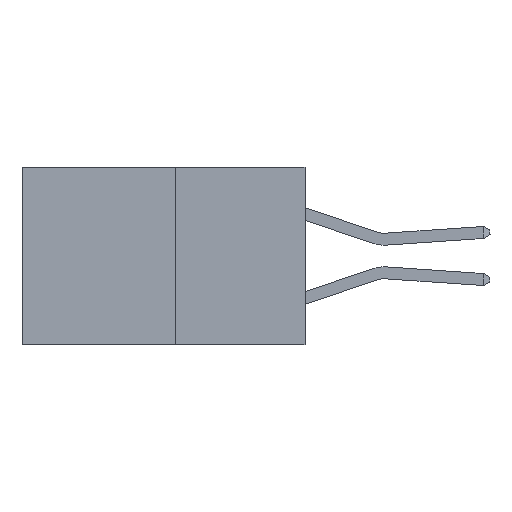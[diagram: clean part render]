
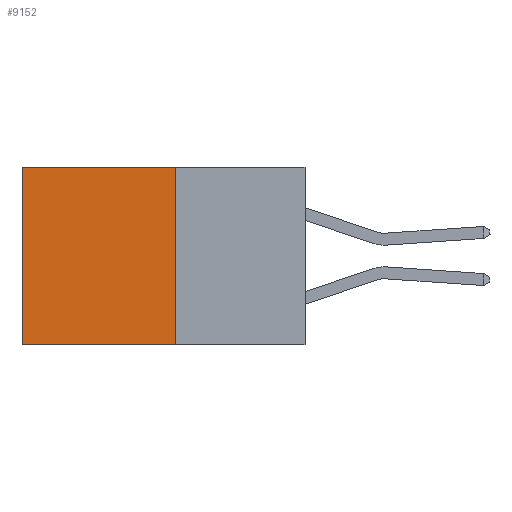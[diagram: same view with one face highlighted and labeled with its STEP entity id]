
A CAD part, left-side view. The second image highlights one B-rep face of the part: STEP entity #9152.
In plain terms, the highlighted planar face has unit normal (-1, 0, 0).
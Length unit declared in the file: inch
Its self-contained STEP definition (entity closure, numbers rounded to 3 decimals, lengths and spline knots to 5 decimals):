
#1104 = DIRECTION ( 'NONE',  ( 0., 0., -1. ) ) ;
#1160 = CARTESIAN_POINT ( 'NONE',  ( 0.277, 0.59, -0.37 ) ) ;
#1604 = ORIENTED_EDGE ( 'NONE', *, *, #6473, .T. ) ;
#3085 = CARTESIAN_POINT ( 'NONE',  ( 0.277, 0.59, -0.37 ) ) ;
#3166 = VECTOR ( 'NONE', #11362, 39.37008 ) ;
#3764 = AXIS2_PLACEMENT_3D ( 'NONE', #15248, #8319, #1104 ) ;
#4315 = VECTOR ( 'NONE', #7587, 39.37008 ) ;
#4835 = VERTEX_POINT ( 'NONE', #8728 ) ;
#4884 = EDGE_CURVE ( 'NONE', #4835, #9971, #13281, .T. ) ;
#5277 = VERTEX_POINT ( 'NONE', #1160 ) ;
#5407 = LINE ( 'NONE', #7884, #7765 ) ;
#5604 = VECTOR ( 'NONE', #14549, 39.37008 ) ;
#5704 = EDGE_CURVE ( 'NONE', #9971, #5277, #14861, .T. ) ;
#6037 = LINE ( 'NONE', #3085, #3166 ) ;
#6473 = EDGE_CURVE ( 'NONE', #4835, #12901, #5407, .T. ) ;
#7451 = CARTESIAN_POINT ( 'NONE',  ( 0.277, 0.27, -0.37 ) ) ;
#7587 = DIRECTION ( 'NONE',  ( 0., 0., -1. ) ) ;
#7765 = VECTOR ( 'NONE', #12518, 39.37008 ) ;
#7884 = CARTESIAN_POINT ( 'NONE',  ( 0.277, 0.27, 0. ) ) ;
#8319 = DIRECTION ( 'NONE',  ( 1., 0., 0. ) ) ;
#8702 = CARTESIAN_POINT ( 'NONE',  ( 0.277, 0.27, -0.37 ) ) ;
#8728 = CARTESIAN_POINT ( 'NONE',  ( 0.277, 0.27, 0. ) ) ;
#9152 = ADVANCED_FACE ( 'NONE', ( #10611 ), #12956, .F. ) ;
#9971 = VERTEX_POINT ( 'NONE', #8702 ) ;
#10003 = ORIENTED_EDGE ( 'NONE', *, *, #4884, .F. ) ;
#10611 = FACE_OUTER_BOUND ( 'NONE', #13956, .T. ) ;
#11362 = DIRECTION ( 'NONE',  ( 0., 0., -1. ) ) ;
#11679 = ORIENTED_EDGE ( 'NONE', *, *, #12272, .T. ) ;
#12231 = CARTESIAN_POINT ( 'NONE',  ( 0.277, 0.27, -0.37 ) ) ;
#12272 = EDGE_CURVE ( 'NONE', #12901, #5277, #6037, .T. ) ;
#12518 = DIRECTION ( 'NONE',  ( 0., 1., 0. ) ) ;
#12901 = VERTEX_POINT ( 'NONE', #13640 ) ;
#12956 = PLANE ( 'NONE',  #3764 ) ;
#13281 = LINE ( 'NONE', #7451, #4315 ) ;
#13627 = ORIENTED_EDGE ( 'NONE', *, *, #5704, .F. ) ;
#13640 = CARTESIAN_POINT ( 'NONE',  ( 0.277, 0.59, 0. ) ) ;
#13956 = EDGE_LOOP ( 'NONE', ( #11679, #13627, #10003, #1604 ) ) ;
#14549 = DIRECTION ( 'NONE',  ( 0., 1., 0. ) ) ;
#14861 = LINE ( 'NONE', #12231, #5604 ) ;
#15248 = CARTESIAN_POINT ( 'NONE',  ( 0.277, 0.27, -0.37 ) ) ;
